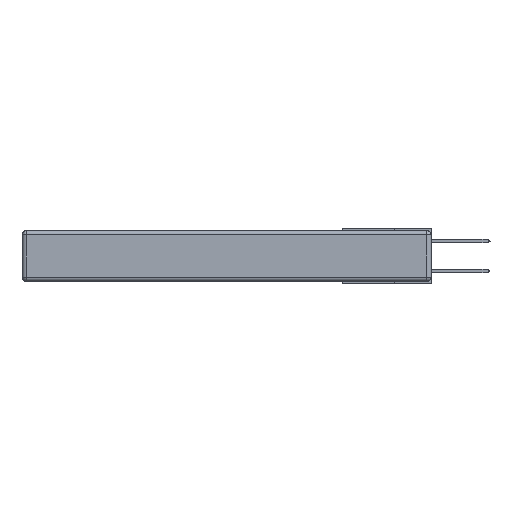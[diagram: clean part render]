
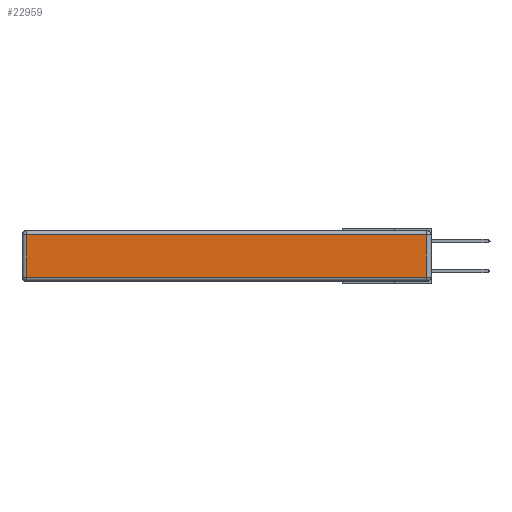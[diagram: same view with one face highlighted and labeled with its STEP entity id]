
A CAD part, left-side view. The second image highlights one B-rep face of the part: STEP entity #22959.
In plain terms, the highlighted planar face has unit normal (-1, 0, 0).
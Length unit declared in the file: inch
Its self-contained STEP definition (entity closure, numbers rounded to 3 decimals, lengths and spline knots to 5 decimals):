
#279 = VECTOR ( 'NONE', #9613, 39.37008 ) ;
#872 = LINE ( 'NONE', #8115, #26994 ) ;
#1079 = CARTESIAN_POINT ( 'NONE',  ( 0., 0.03, -0.313 ) ) ;
#1769 = DIRECTION ( 'NONE',  ( -1., 0., 0. ) ) ;
#6318 = FACE_OUTER_BOUND ( 'NONE', #8918, .T. ) ;
#6434 = CARTESIAN_POINT ( 'NONE',  ( 0., 0.03, -0.03 ) ) ;
#6528 = VERTEX_POINT ( 'NONE', #1079 ) ;
#8115 = CARTESIAN_POINT ( 'NONE',  ( 0., 2.75, -0.03 ) ) ;
#8918 = EDGE_LOOP ( 'NONE', ( #18658, #14898, #26869, #17126 ) ) ;
#9613 = DIRECTION ( 'NONE',  ( 0., 0., 1. ) ) ;
#9637 = LINE ( 'NONE', #18242, #24188 ) ;
#12120 = VECTOR ( 'NONE', #26423, 39.37008 ) ;
#12473 = VERTEX_POINT ( 'NONE', #30695 ) ;
#14365 = EDGE_CURVE ( 'NONE', #12473, #18764, #9637, .T. ) ;
#14898 = ORIENTED_EDGE ( 'NONE', *, *, #24377, .T. ) ;
#15077 = LINE ( 'NONE', #28198, #12120 ) ;
#15752 = EDGE_CURVE ( 'NONE', #18764, #6528, #15077, .T. ) ;
#15986 = PLANE ( 'NONE',  #22840 ) ;
#17126 = ORIENTED_EDGE ( 'NONE', *, *, #14365, .T. ) ;
#17928 = DIRECTION ( 'NONE',  ( 0., 0., -1. ) ) ;
#18242 = CARTESIAN_POINT ( 'NONE',  ( 0., 2.72, -0.343 ) ) ;
#18387 = DIRECTION ( 'NONE',  ( 0., 0., 1. ) ) ;
#18658 = ORIENTED_EDGE ( 'NONE', *, *, #15752, .T. ) ;
#18698 = CARTESIAN_POINT ( 'NONE',  ( 0., 0., -0.343 ) ) ;
#18764 = VERTEX_POINT ( 'NONE', #23963 ) ;
#20799 = LINE ( 'NONE', #26419, #279 ) ;
#22840 = AXIS2_PLACEMENT_3D ( 'NONE', #18698, #1769, #18387 ) ;
#22959 = ADVANCED_FACE ( 'NONE', ( #6318 ), #15986, .T. ) ;
#23963 = CARTESIAN_POINT ( 'NONE',  ( 0., 2.72, -0.313 ) ) ;
#24188 = VECTOR ( 'NONE', #17928, 39.37008 ) ;
#24377 = EDGE_CURVE ( 'NONE', #6528, #28974, #20799, .T. ) ;
#26419 = CARTESIAN_POINT ( 'NONE',  ( 0., 0.03, -0.343 ) ) ;
#26423 = DIRECTION ( 'NONE',  ( 0., -1., 0. ) ) ;
#26869 = ORIENTED_EDGE ( 'NONE', *, *, #28379, .T. ) ;
#26994 = VECTOR ( 'NONE', #29706, 39.37008 ) ;
#28198 = CARTESIAN_POINT ( 'NONE',  ( 0., 0., -0.313 ) ) ;
#28379 = EDGE_CURVE ( 'NONE', #28974, #12473, #872, .T. ) ;
#28974 = VERTEX_POINT ( 'NONE', #6434 ) ;
#29706 = DIRECTION ( 'NONE',  ( 0., 1., 0. ) ) ;
#30695 = CARTESIAN_POINT ( 'NONE',  ( 0., 2.72, -0.03 ) ) ;
